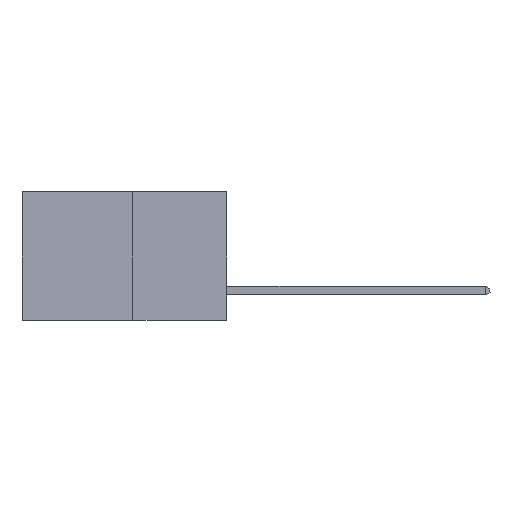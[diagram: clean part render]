
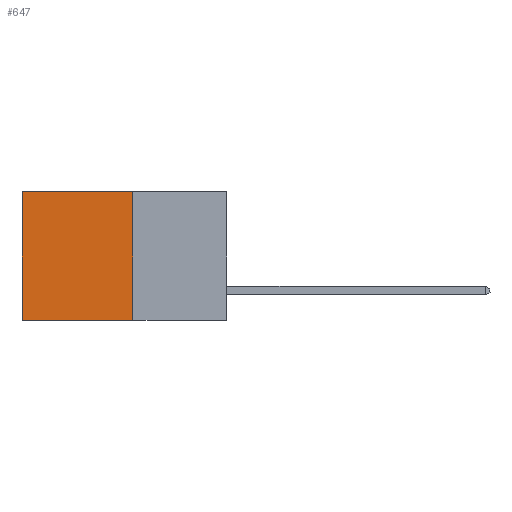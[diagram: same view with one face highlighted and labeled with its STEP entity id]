
A CAD part, left-side view. The second image highlights one B-rep face of the part: STEP entity #647.
In plain terms, the highlighted planar face has unit normal (-1, 0, 0).
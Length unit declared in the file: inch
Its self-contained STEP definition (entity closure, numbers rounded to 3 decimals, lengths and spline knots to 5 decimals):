
#647 = ADVANCED_FACE ( 'NONE', ( #892 ), #3958, .F. ) ;
#892 = FACE_OUTER_BOUND ( 'NONE', #902, .T. ) ;
#902 = EDGE_LOOP ( 'NONE', ( #3549, #8238, #6451, #6742 ) ) ;
#978 = EDGE_CURVE ( 'NONE', #6704, #10833, #8885, .T. ) ;
#991 = DIRECTION ( 'NONE',  ( 1., 0., 0. ) ) ;
#1010 = CARTESIAN_POINT ( 'NONE',  ( 0.277, 0.27, -0.37 ) ) ;
#1012 = DIRECTION ( 'NONE',  ( 0., 0., -1. ) ) ;
#1286 = DIRECTION ( 'NONE',  ( 0., 0., -1. ) ) ;
#1531 = VERTEX_POINT ( 'NONE', #6974 ) ;
#1877 = VECTOR ( 'NONE', #3580, 39.37008 ) ;
#3236 = CARTESIAN_POINT ( 'NONE',  ( 0.277, 0.27, -0.37 ) ) ;
#3549 = ORIENTED_EDGE ( 'NONE', *, *, #9698, .T. ) ;
#3580 = DIRECTION ( 'NONE',  ( 0., 0., -1. ) ) ;
#3875 = CARTESIAN_POINT ( 'NONE',  ( 0.277, 0.59, -0.37 ) ) ;
#3958 = PLANE ( 'NONE',  #9707 ) ;
#5465 = VECTOR ( 'NONE', #1286, 39.37008 ) ;
#5819 = LINE ( 'NONE', #7789, #10232 ) ;
#6278 = VERTEX_POINT ( 'NONE', #8334 ) ;
#6451 = ORIENTED_EDGE ( 'NONE', *, *, #9138, .F. ) ;
#6704 = VERTEX_POINT ( 'NONE', #9423 ) ;
#6742 = ORIENTED_EDGE ( 'NONE', *, *, #11339, .T. ) ;
#6974 = CARTESIAN_POINT ( 'NONE',  ( 0.277, 0.59, 0. ) ) ;
#7789 = CARTESIAN_POINT ( 'NONE',  ( 0.277, 0.27, 0. ) ) ;
#7989 = CARTESIAN_POINT ( 'NONE',  ( 0.277, 0.59, -0.37 ) ) ;
#8101 = LINE ( 'NONE', #3236, #5465 ) ;
#8238 = ORIENTED_EDGE ( 'NONE', *, *, #978, .F. ) ;
#8334 = CARTESIAN_POINT ( 'NONE',  ( 0.277, 0.27, 0. ) ) ;
#8664 = DIRECTION ( 'NONE',  ( 0., 1., 0. ) ) ;
#8885 = LINE ( 'NONE', #11490, #11144 ) ;
#9048 = LINE ( 'NONE', #7989, #1877 ) ;
#9138 = EDGE_CURVE ( 'NONE', #6278, #6704, #8101, .T. ) ;
#9423 = CARTESIAN_POINT ( 'NONE',  ( 0.277, 0.27, -0.37 ) ) ;
#9698 = EDGE_CURVE ( 'NONE', #1531, #10833, #9048, .T. ) ;
#9707 = AXIS2_PLACEMENT_3D ( 'NONE', #1010, #991, #1012 ) ;
#10232 = VECTOR ( 'NONE', #8664, 39.37008 ) ;
#10493 = DIRECTION ( 'NONE',  ( 0., 1., 0. ) ) ;
#10833 = VERTEX_POINT ( 'NONE', #3875 ) ;
#11144 = VECTOR ( 'NONE', #10493, 39.37008 ) ;
#11339 = EDGE_CURVE ( 'NONE', #6278, #1531, #5819, .T. ) ;
#11490 = CARTESIAN_POINT ( 'NONE',  ( 0.277, 0.27, -0.37 ) ) ;
